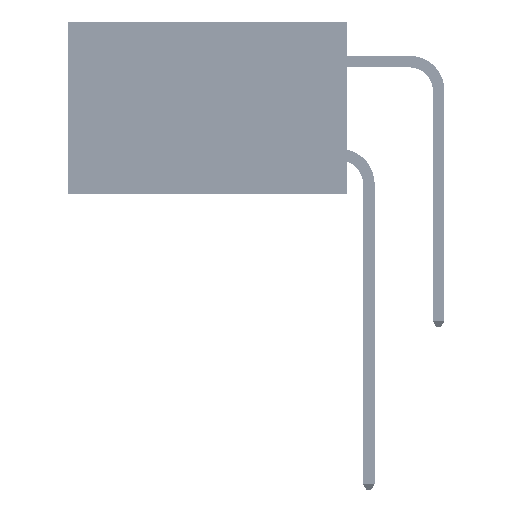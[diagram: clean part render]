
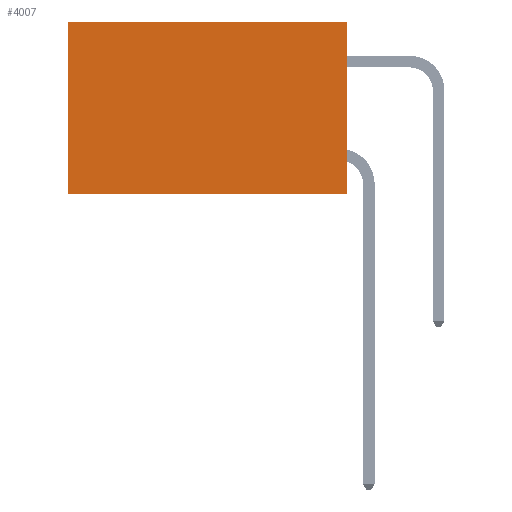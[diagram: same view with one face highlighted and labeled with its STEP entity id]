
A CAD part, left-side view. The second image highlights one B-rep face of the part: STEP entity #4007.
In plain terms, the highlighted planar face has unit normal (-1, 0, 0).
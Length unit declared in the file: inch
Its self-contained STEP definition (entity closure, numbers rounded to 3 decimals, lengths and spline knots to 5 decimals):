
#1765 = VECTOR ( 'NONE', #10637, 39.37008 ) ;
#1913 = CARTESIAN_POINT ( 'NONE',  ( 0.2875, 0., 0. ) ) ;
#2357 = DIRECTION ( 'NONE',  ( 0., 1., 0. ) ) ;
#2776 = EDGE_CURVE ( 'NONE', #31476, #21802, #21043, .T. ) ;
#3659 = EDGE_CURVE ( 'NONE', #21802, #39647, #23662, .T. ) ;
#4007 = ADVANCED_FACE ( 'NONE', ( #46062 ), #39111, .F. ) ;
#4515 = EDGE_CURVE ( 'NONE', #31476, #7619, #33190, .T. ) ;
#6012 = CARTESIAN_POINT ( 'NONE',  ( 0.2875, 0., -0.37 ) ) ;
#6506 = LINE ( 'NONE', #6012, #24659 ) ;
#7143 = CARTESIAN_POINT ( 'NONE',  ( 0.2875, 0., 0. ) ) ;
#7619 = VERTEX_POINT ( 'NONE', #29658 ) ;
#10203 = EDGE_LOOP ( 'NONE', ( #19656, #45422, #31602, #14499 ) ) ;
#10637 = DIRECTION ( 'NONE',  ( 0., 1., 0. ) ) ;
#11689 = CARTESIAN_POINT ( 'NONE',  ( 0.2875, 0.6, -0.37 ) ) ;
#11990 = CARTESIAN_POINT ( 'NONE',  ( 0.2875, 0.6, 0. ) ) ;
#13145 = CARTESIAN_POINT ( 'NONE',  ( 0.2875, 0., 0. ) ) ;
#14338 = EDGE_CURVE ( 'NONE', #7619, #39647, #6506, .T. ) ;
#14499 = ORIENTED_EDGE ( 'NONE', *, *, #2776, .T. ) ;
#19656 = ORIENTED_EDGE ( 'NONE', *, *, #3659, .T. ) ;
#21043 = LINE ( 'NONE', #7143, #1765 ) ;
#21145 = DIRECTION ( 'NONE',  ( 0., 0., -1. ) ) ;
#21802 = VERTEX_POINT ( 'NONE', #34820 ) ;
#23570 = VECTOR ( 'NONE', #38135, 39.37008 ) ;
#23662 = LINE ( 'NONE', #11990, #41638 ) ;
#24659 = VECTOR ( 'NONE', #2357, 39.37008 ) ;
#29658 = CARTESIAN_POINT ( 'NONE',  ( 0.2875, 0., -0.37 ) ) ;
#31476 = VERTEX_POINT ( 'NONE', #13145 ) ;
#31602 = ORIENTED_EDGE ( 'NONE', *, *, #4515, .F. ) ;
#33190 = LINE ( 'NONE', #1913, #23570 ) ;
#34820 = CARTESIAN_POINT ( 'NONE',  ( 0.2875, 0.6, 0. ) ) ;
#34919 = AXIS2_PLACEMENT_3D ( 'NONE', #46104, #42694, #21145 ) ;
#38135 = DIRECTION ( 'NONE',  ( 0., 0., -1. ) ) ;
#39111 = PLANE ( 'NONE',  #34919 ) ;
#39647 = VERTEX_POINT ( 'NONE', #11689 ) ;
#40859 = DIRECTION ( 'NONE',  ( 0., 0., -1. ) ) ;
#41638 = VECTOR ( 'NONE', #40859, 39.37008 ) ;
#42694 = DIRECTION ( 'NONE',  ( 1., 0., 0. ) ) ;
#45422 = ORIENTED_EDGE ( 'NONE', *, *, #14338, .F. ) ;
#46062 = FACE_OUTER_BOUND ( 'NONE', #10203, .T. ) ;
#46104 = CARTESIAN_POINT ( 'NONE',  ( 0.2875, 0., 0. ) ) ;
